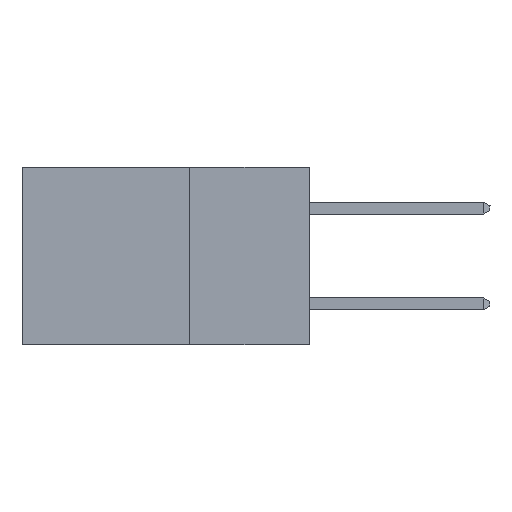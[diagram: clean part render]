
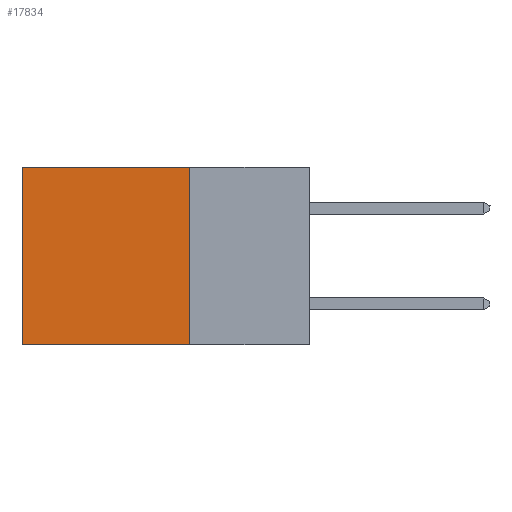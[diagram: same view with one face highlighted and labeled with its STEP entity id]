
A CAD part, left-side view. The second image highlights one B-rep face of the part: STEP entity #17834.
In plain terms, the highlighted planar face has unit normal (-1, 0, 0).
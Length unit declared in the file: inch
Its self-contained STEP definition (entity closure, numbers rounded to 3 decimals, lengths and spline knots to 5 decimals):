
#968 = EDGE_CURVE ( 'NONE', #12536, #10646, #18550, .T. ) ;
#1042 = EDGE_CURVE ( 'NONE', #15441, #12536, #12919, .T. ) ;
#1712 = CARTESIAN_POINT ( 'NONE',  ( 0.2875, 0.25, -0.37 ) ) ;
#2355 = VECTOR ( 'NONE', #25116, 39.37008 ) ;
#3582 = CARTESIAN_POINT ( 'NONE',  ( 0.2875, 0.25, 0. ) ) ;
#4070 = LINE ( 'NONE', #1712, #16431 ) ;
#5997 = VECTOR ( 'NONE', #22406, 39.37008 ) ;
#8312 = CARTESIAN_POINT ( 'NONE',  ( 0.2875, 0.25, 0. ) ) ;
#8505 = CARTESIAN_POINT ( 'NONE',  ( 0.2875, 0.25, -0.37 ) ) ;
#8613 = PLANE ( 'NONE',  #26593 ) ;
#8747 = ORIENTED_EDGE ( 'NONE', *, *, #21066, .F. ) ;
#9887 = VERTEX_POINT ( 'NONE', #8505 ) ;
#10646 = VERTEX_POINT ( 'NONE', #17003 ) ;
#11247 = DIRECTION ( 'NONE',  ( 0., 1., 0. ) ) ;
#12536 = VERTEX_POINT ( 'NONE', #13068 ) ;
#12919 = LINE ( 'NONE', #29580, #5997 ) ;
#13068 = CARTESIAN_POINT ( 'NONE',  ( 0.2875, 0.6, 0. ) ) ;
#13295 = LINE ( 'NONE', #8312, #2355 ) ;
#13901 = DIRECTION ( 'NONE',  ( 0., 0., -1. ) ) ;
#15040 = ORIENTED_EDGE ( 'NONE', *, *, #25362, .F. ) ;
#15441 = VERTEX_POINT ( 'NONE', #3582 ) ;
#16375 = ORIENTED_EDGE ( 'NONE', *, *, #1042, .T. ) ;
#16431 = VECTOR ( 'NONE', #11247, 39.37008 ) ;
#16523 = CARTESIAN_POINT ( 'NONE',  ( 0.2875, 0.6, 0. ) ) ;
#17003 = CARTESIAN_POINT ( 'NONE',  ( 0.2875, 0.6, -0.37 ) ) ;
#17834 = ADVANCED_FACE ( 'NONE', ( #25109 ), #8613, .F. ) ;
#17955 = DIRECTION ( 'NONE',  ( 1., 0., 0. ) ) ;
#18550 = LINE ( 'NONE', #16523, #19915 ) ;
#19915 = VECTOR ( 'NONE', #13901, 39.37008 ) ;
#21066 = EDGE_CURVE ( 'NONE', #15441, #9887, #13295, .T. ) ;
#22406 = DIRECTION ( 'NONE',  ( 0., 1., 0. ) ) ;
#22932 = CARTESIAN_POINT ( 'NONE',  ( 0.2875, 0.25, 0. ) ) ;
#23922 = EDGE_LOOP ( 'NONE', ( #27074, #15040, #8747, #16375 ) ) ;
#25109 = FACE_OUTER_BOUND ( 'NONE', #23922, .T. ) ;
#25116 = DIRECTION ( 'NONE',  ( 0., 0., -1. ) ) ;
#25362 = EDGE_CURVE ( 'NONE', #9887, #10646, #4070, .T. ) ;
#26593 = AXIS2_PLACEMENT_3D ( 'NONE', #22932, #17955, #27605 ) ;
#27074 = ORIENTED_EDGE ( 'NONE', *, *, #968, .T. ) ;
#27605 = DIRECTION ( 'NONE',  ( 0., 0., -1. ) ) ;
#29580 = CARTESIAN_POINT ( 'NONE',  ( 0.2875, 0.25, 0. ) ) ;
